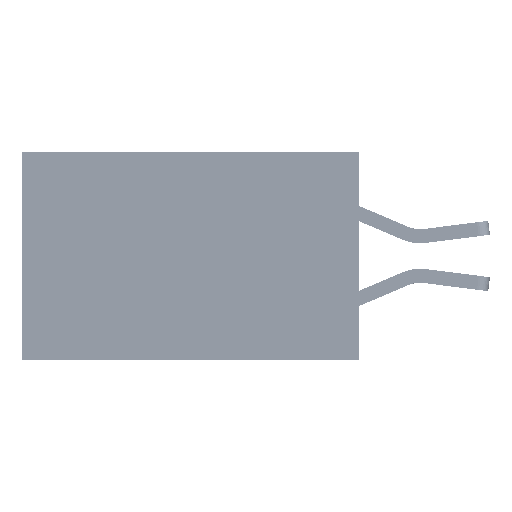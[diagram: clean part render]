
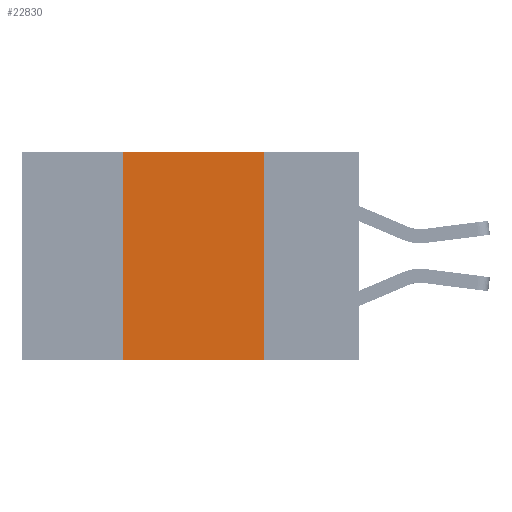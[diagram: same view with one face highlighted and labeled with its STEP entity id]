
A CAD part, left-side view. The second image highlights one B-rep face of the part: STEP entity #22830.
In plain terms, the highlighted planar face has unit normal (-1, 0, 0).
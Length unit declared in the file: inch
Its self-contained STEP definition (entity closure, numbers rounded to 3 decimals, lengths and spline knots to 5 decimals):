
#1035 = ORIENTED_EDGE ( 'NONE', *, *, #8305, .F. ) ;
#1089 = EDGE_LOOP ( 'NONE', ( #13531, #1035, #3733, #40063 ) ) ;
#2404 = DIRECTION ( 'NONE',  ( 0., 0., -1. ) ) ;
#3461 = VECTOR ( 'NONE', #2404, 39.37008 ) ;
#3733 = ORIENTED_EDGE ( 'NONE', *, *, #19938, .F. ) ;
#6260 = LINE ( 'NONE', #47941, #42622 ) ;
#8305 = EDGE_CURVE ( 'NONE', #29766, #36627, #6260, .T. ) ;
#8331 = LINE ( 'NONE', #39393, #43486 ) ;
#8412 = PLANE ( 'NONE',  #24132 ) ;
#8922 = EDGE_CURVE ( 'NONE', #36627, #34030, #27091, .T. ) ;
#13420 = CARTESIAN_POINT ( 'NONE',  ( 0., 0.17, 0. ) ) ;
#13531 = ORIENTED_EDGE ( 'NONE', *, *, #8922, .F. ) ;
#17094 = CARTESIAN_POINT ( 'NONE',  ( 0., 0.17, -0.37 ) ) ;
#17431 = DIRECTION ( 'NONE',  ( 0., 0., 1. ) ) ;
#18554 = VECTOR ( 'NONE', #17431, 39.37008 ) ;
#19938 = EDGE_CURVE ( 'NONE', #49731, #29766, #28893, .T. ) ;
#20214 = DIRECTION ( 'NONE',  ( 1., 0., 0. ) ) ;
#20723 = DIRECTION ( 'NONE',  ( 0., 0., -1. ) ) ;
#22830 = ADVANCED_FACE ( 'NONE', ( #40683 ), #8412, .F. ) ;
#24132 = AXIS2_PLACEMENT_3D ( 'NONE', #35172, #20214, #20723 ) ;
#24147 = DIRECTION ( 'NONE',  ( 0., -1., 0. ) ) ;
#25841 = CARTESIAN_POINT ( 'NONE',  ( 0., 0.42, -0.37 ) ) ;
#27091 = LINE ( 'NONE', #13420, #3461 ) ;
#28893 = LINE ( 'NONE', #40651, #18554 ) ;
#29491 = EDGE_CURVE ( 'NONE', #49731, #34030, #8331, .T. ) ;
#29766 = VERTEX_POINT ( 'NONE', #36695 ) ;
#34030 = VERTEX_POINT ( 'NONE', #17094 ) ;
#35172 = CARTESIAN_POINT ( 'NONE',  ( 0., 0.6, 0. ) ) ;
#35539 = CARTESIAN_POINT ( 'NONE',  ( 0., 0.17, 0. ) ) ;
#36627 = VERTEX_POINT ( 'NONE', #35539 ) ;
#36695 = CARTESIAN_POINT ( 'NONE',  ( 0., 0.42, 0. ) ) ;
#39393 = CARTESIAN_POINT ( 'NONE',  ( 0., 0.6, -0.37 ) ) ;
#40063 = ORIENTED_EDGE ( 'NONE', *, *, #29491, .T. ) ;
#40642 = DIRECTION ( 'NONE',  ( 0., -1., 0. ) ) ;
#40651 = CARTESIAN_POINT ( 'NONE',  ( 0., 0.42, 0. ) ) ;
#40683 = FACE_OUTER_BOUND ( 'NONE', #1089, .T. ) ;
#42622 = VECTOR ( 'NONE', #40642, 39.37008 ) ;
#43486 = VECTOR ( 'NONE', #24147, 39.37008 ) ;
#47941 = CARTESIAN_POINT ( 'NONE',  ( 0., 0.6, 0. ) ) ;
#49731 = VERTEX_POINT ( 'NONE', #25841 ) ;
